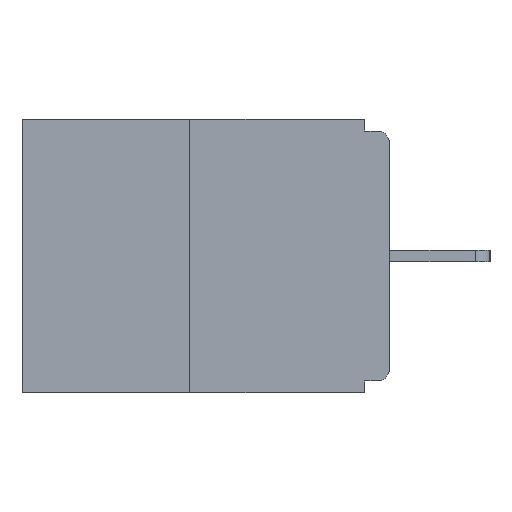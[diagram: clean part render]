
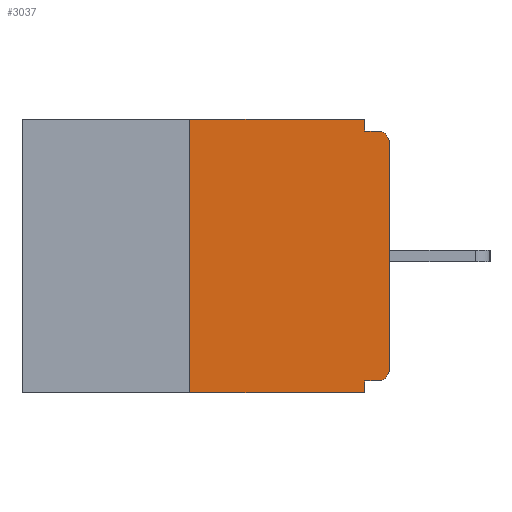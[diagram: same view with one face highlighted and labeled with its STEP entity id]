
A CAD part, left-side view. The second image highlights one B-rep face of the part: STEP entity #3037.
In plain terms, the highlighted planar face has unit normal (-1, 0, 0).
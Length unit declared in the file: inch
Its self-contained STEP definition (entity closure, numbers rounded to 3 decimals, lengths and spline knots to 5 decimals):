
#348 = CARTESIAN_POINT ( 'NONE',  ( 0., 0.015, -0.313 ) ) ;
#357 = CARTESIAN_POINT ( 'NONE',  ( 0., 0., -0.015 ) ) ;
#904 = DIRECTION ( 'NONE',  ( 0., 0., -1. ) ) ;
#1100 = EDGE_CURVE ( 'NONE', #21859, #18206, #20485, .T. ) ;
#2570 = LINE ( 'NONE', #19373, #16607 ) ;
#3037 = ADVANCED_FACE ( 'NONE', ( #5216 ), #13819, .F. ) ;
#3108 = DIRECTION ( 'NONE',  ( 1., 0., 0. ) ) ;
#3347 = VERTEX_POINT ( 'NONE', #24054 ) ;
#3570 = CARTESIAN_POINT ( 'NONE',  ( 0., 0.015, -0.03 ) ) ;
#3755 = ORIENTED_EDGE ( 'NONE', *, *, #9044, .F. ) ;
#4051 = ORIENTED_EDGE ( 'NONE', *, *, #1100, .T. ) ;
#4602 = CARTESIAN_POINT ( 'NONE',  ( 0., 0.25, 0. ) ) ;
#4603 = VERTEX_POINT ( 'NONE', #4602 ) ;
#4635 = CARTESIAN_POINT ( 'NONE',  ( 0., 0.25, 0. ) ) ;
#4904 = VECTOR ( 'NONE', #17133, 39.37008 ) ;
#5216 = FACE_OUTER_BOUND ( 'NONE', #27273, .T. ) ;
#5235 = LINE ( 'NONE', #23981, #27450 ) ;
#7764 = ORIENTED_EDGE ( 'NONE', *, *, #13828, .T. ) ;
#8434 = CARTESIAN_POINT ( 'NONE',  ( 0., 0.25, -0.343 ) ) ;
#8564 = EDGE_CURVE ( 'NONE', #14064, #3347, #18874, .T. ) ;
#8608 = EDGE_CURVE ( 'NONE', #3347, #27178, #25821, .T. ) ;
#8904 = ORIENTED_EDGE ( 'NONE', *, *, #8564, .F. ) ;
#9044 = EDGE_CURVE ( 'NONE', #4603, #14064, #2570, .T. ) ;
#9164 = AXIS2_PLACEMENT_3D ( 'NONE', #3570, #13722, #904 ) ;
#9875 = CARTESIAN_POINT ( 'NONE',  ( 0., 0.015, -0.015 ) ) ;
#10295 = DIRECTION ( 'NONE',  ( 0., 0., 1. ) ) ;
#10595 = EDGE_CURVE ( 'NONE', #16086, #27178, #13584, .T. ) ;
#10859 = ORIENTED_EDGE ( 'NONE', *, *, #17877, .F. ) ;
#11600 = DIRECTION ( 'NONE',  ( 0., 0., -1. ) ) ;
#11811 = CARTESIAN_POINT ( 'NONE',  ( 0., 0., 0. ) ) ;
#12916 = VERTEX_POINT ( 'NONE', #17013 ) ;
#13453 = DIRECTION ( 'NONE',  ( 0., 1., 0. ) ) ;
#13584 = CIRCLE ( 'NONE', #9164, 0.015 ) ;
#13688 = CARTESIAN_POINT ( 'NONE',  ( 0., 0.46, 0. ) ) ;
#13722 = DIRECTION ( 'NONE',  ( -1., 0., 0. ) ) ;
#13819 = PLANE ( 'NONE',  #25644 ) ;
#13828 = EDGE_CURVE ( 'NONE', #14745, #16086, #20690, .T. ) ;
#14064 = VERTEX_POINT ( 'NONE', #14606 ) ;
#14134 = VECTOR ( 'NONE', #19541, 39.37008 ) ;
#14215 = VECTOR ( 'NONE', #16410, 39.37008 ) ;
#14253 = CIRCLE ( 'NONE', #22219, 0.015 ) ;
#14606 = CARTESIAN_POINT ( 'NONE',  ( 0., 0.031, 0. ) ) ;
#14708 = EDGE_CURVE ( 'NONE', #12916, #24479, #5235, .T. ) ;
#14745 = VERTEX_POINT ( 'NONE', #26219 ) ;
#14759 = CARTESIAN_POINT ( 'NONE',  ( 0., 0.031, -0.343 ) ) ;
#14848 = CARTESIAN_POINT ( 'NONE',  ( 0., 0.031, 0. ) ) ;
#14942 = CARTESIAN_POINT ( 'NONE',  ( 0., 0.031, -0.328 ) ) ;
#15195 = LINE ( 'NONE', #4635, #4904 ) ;
#16076 = EDGE_CURVE ( 'NONE', #21859, #4603, #15195, .T. ) ;
#16086 = VERTEX_POINT ( 'NONE', #25617 ) ;
#16410 = DIRECTION ( 'NONE',  ( 0., 0., -1. ) ) ;
#16426 = VECTOR ( 'NONE', #27347, 39.37008 ) ;
#16607 = VECTOR ( 'NONE', #23557, 39.37008 ) ;
#17013 = CARTESIAN_POINT ( 'NONE',  ( 0., 0.015, -0.328 ) ) ;
#17133 = DIRECTION ( 'NONE',  ( 0., 0., 1. ) ) ;
#17877 = EDGE_CURVE ( 'NONE', #24479, #18206, #24765, .T. ) ;
#18124 = CARTESIAN_POINT ( 'NONE',  ( 0., 0.46, -0.343 ) ) ;
#18206 = VERTEX_POINT ( 'NONE', #14759 ) ;
#18874 = LINE ( 'NONE', #14848, #16426 ) ;
#19003 = DIRECTION ( 'NONE',  ( -1., 0., 0. ) ) ;
#19373 = CARTESIAN_POINT ( 'NONE',  ( 0., 0.46, 0. ) ) ;
#19467 = ORIENTED_EDGE ( 'NONE', *, *, #8608, .F. ) ;
#19531 = ORIENTED_EDGE ( 'NONE', *, *, #10595, .T. ) ;
#19541 = DIRECTION ( 'NONE',  ( 0., -1., 0. ) ) ;
#20393 = ORIENTED_EDGE ( 'NONE', *, *, #25377, .T. ) ;
#20485 = LINE ( 'NONE', #18124, #24844 ) ;
#20690 = LINE ( 'NONE', #11811, #26094 ) ;
#21859 = VERTEX_POINT ( 'NONE', #8434 ) ;
#22219 = AXIS2_PLACEMENT_3D ( 'NONE', #348, #19003, #23444 ) ;
#23444 = DIRECTION ( 'NONE',  ( 0., 0., -1. ) ) ;
#23557 = DIRECTION ( 'NONE',  ( 0., -1., 0. ) ) ;
#23981 = CARTESIAN_POINT ( 'NONE',  ( 0., 0., -0.328 ) ) ;
#24054 = CARTESIAN_POINT ( 'NONE',  ( 0., 0.031, -0.015 ) ) ;
#24209 = ORIENTED_EDGE ( 'NONE', *, *, #16076, .F. ) ;
#24479 = VERTEX_POINT ( 'NONE', #14942 ) ;
#24765 = LINE ( 'NONE', #26698, #14215 ) ;
#24844 = VECTOR ( 'NONE', #27169, 39.37008 ) ;
#25377 = EDGE_CURVE ( 'NONE', #12916, #14745, #14253, .T. ) ;
#25617 = CARTESIAN_POINT ( 'NONE',  ( 0., 0., -0.03 ) ) ;
#25644 = AXIS2_PLACEMENT_3D ( 'NONE', #13688, #3108, #11600 ) ;
#25821 = LINE ( 'NONE', #357, #14134 ) ;
#26094 = VECTOR ( 'NONE', #10295, 39.37008 ) ;
#26219 = CARTESIAN_POINT ( 'NONE',  ( 0., 0., -0.313 ) ) ;
#26698 = CARTESIAN_POINT ( 'NONE',  ( 0., 0.031, -0.343 ) ) ;
#26834 = ORIENTED_EDGE ( 'NONE', *, *, #14708, .F. ) ;
#27169 = DIRECTION ( 'NONE',  ( 0., -1., 0. ) ) ;
#27178 = VERTEX_POINT ( 'NONE', #9875 ) ;
#27273 = EDGE_LOOP ( 'NONE', ( #3755, #24209, #4051, #10859, #26834, #20393, #7764, #19531, #19467, #8904 ) ) ;
#27347 = DIRECTION ( 'NONE',  ( 0., 0., -1. ) ) ;
#27450 = VECTOR ( 'NONE', #13453, 39.37008 ) ;
